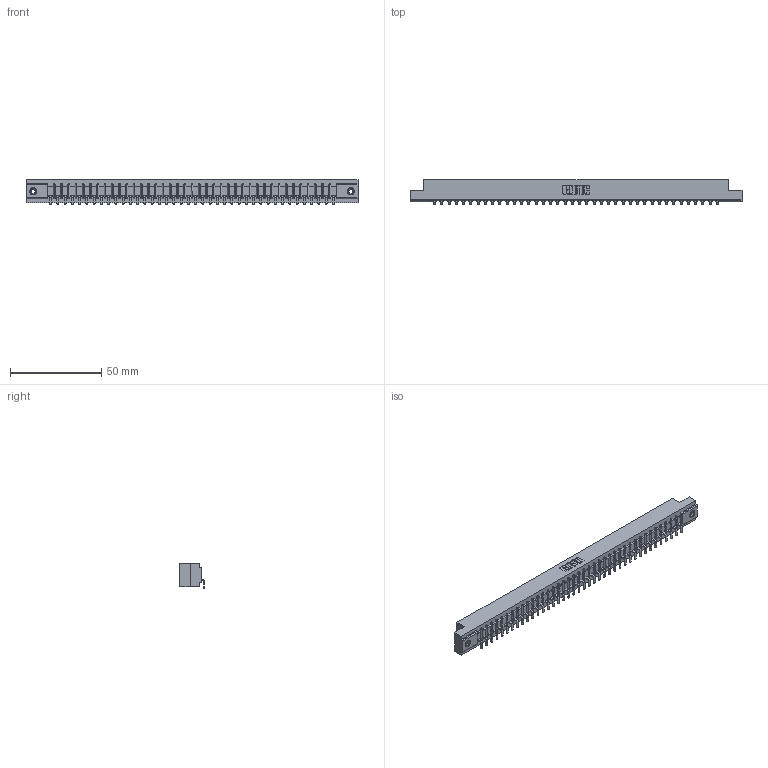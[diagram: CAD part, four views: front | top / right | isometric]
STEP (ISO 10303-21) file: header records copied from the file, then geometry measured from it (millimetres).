
FILE_DESCRIPTION (( 'STEP AP203' ), '1' );
FILE_NAME ('307-040-453-108.STEP', '2020-09-29T10:49:47', ( '' ), ( '' ), 'SwSTEP 2.0', 'SolidWorks 2020', '' );
FILE_SCHEMA (( 'CONFIG_CONTROL_DESIGN' ));
Length unit declared in the file: inch
Products named in the file (4): 307-290-002_553; 345-250-001_345-250-003-102; 307 Part_.156 Dia Mounting Holes; 307-040-453-108
Assembly tree (43 placements, depth 2):
  307-040-453-108
    307 Part_.156 Dia Mounting Holes
    307-290-002_553  x40
    345-250-001_345-250-003-102  x2
Bounding box: 181.51 x 13.32 x 13.5 mm (x, y, z)
Volume: 19402.1 mm3; surface area: 24364.5 mm2
Topology: 43 solids, 43 shells, 3339 faces, 10219 edges, 6694 vertices
Faces by surface type: plane 1982, cylinder 1259, sphere 82, cone 12, torus 4
Entity records: 36577 total; most frequent: CARTESIAN_POINT 6151, ORIENTED_EDGE 6134, DIRECTION 5987, EDGE_CURVE 3067, VECTOR 2347, LINE 2347, VERTEX_POINT 1984, AXIS2_PLACEMENT_3D 1820
